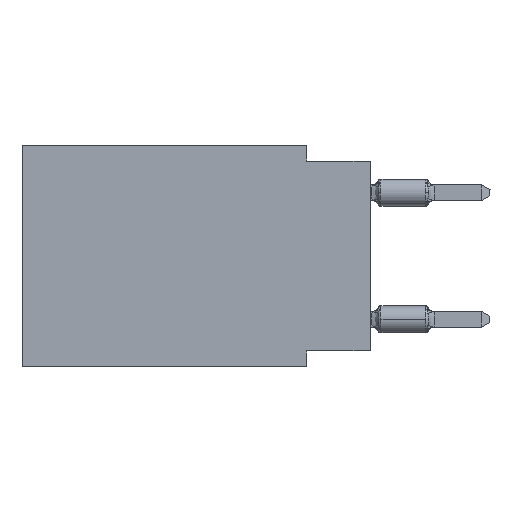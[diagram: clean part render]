
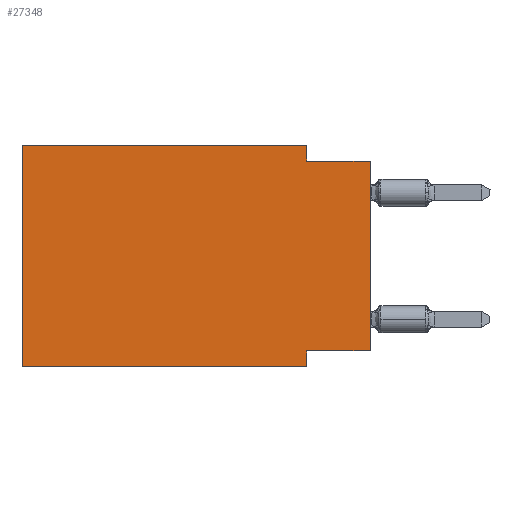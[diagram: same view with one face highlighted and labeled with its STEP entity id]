
A CAD part, left-side view. The second image highlights one B-rep face of the part: STEP entity #27348.
In plain terms, the highlighted planar face has unit normal (-1, 0, 0).
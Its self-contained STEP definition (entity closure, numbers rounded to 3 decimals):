
#410 = CARTESIAN_POINT ( 'NONE',  ( 0., 0., -0.635 ) ) ;
#824 = EDGE_CURVE ( 'NONE', #23125, #20748, #13897, .T. ) ;
#1138 = CARTESIAN_POINT ( 'NONE',  ( 0., 13.97, 0. ) ) ;
#1328 = CARTESIAN_POINT ( 'NONE',  ( 0., 2.54, 0. ) ) ;
#1927 = CARTESIAN_POINT ( 'NONE',  ( 0., 2.54, -0.635 ) ) ;
#3256 = EDGE_CURVE ( 'NONE', #11859, #10257, #14418, .T. ) ;
#3869 = LINE ( 'NONE', #25996, #14602 ) ;
#4015 = VECTOR ( 'NONE', #21537, 1000. ) ;
#4171 = VERTEX_POINT ( 'NONE', #21903 ) ;
#4613 = VECTOR ( 'NONE', #12708, 1000. ) ;
#4654 = CARTESIAN_POINT ( 'NONE',  ( 0., 0., -8.255 ) ) ;
#5295 = VERTEX_POINT ( 'NONE', #4654 ) ;
#5311 = FACE_OUTER_BOUND ( 'NONE', #21102, .T. ) ;
#5463 = LINE ( 'NONE', #19971, #10471 ) ;
#6373 = ORIENTED_EDGE ( 'NONE', *, *, #18525, .F. ) ;
#6732 = CARTESIAN_POINT ( 'NONE',  ( 0., 2.54, 0. ) ) ;
#7529 = DIRECTION ( 'NONE',  ( 0., -1., 0. ) ) ;
#7699 = DIRECTION ( 'NONE',  ( 1., 0., 0. ) ) ;
#8710 = DIRECTION ( 'NONE',  ( 0., 0., 1. ) ) ;
#8904 = LINE ( 'NONE', #17940, #28274 ) ;
#9535 = ORIENTED_EDGE ( 'NONE', *, *, #16182, .F. ) ;
#9789 = VERTEX_POINT ( 'NONE', #6732 ) ;
#10257 = VERTEX_POINT ( 'NONE', #22142 ) ;
#10335 = AXIS2_PLACEMENT_3D ( 'NONE', #1138, #7699, #16742 ) ;
#10471 = VECTOR ( 'NONE', #8710, 1000. ) ;
#10557 = LINE ( 'NONE', #1328, #25677 ) ;
#11704 = EDGE_CURVE ( 'NONE', #9789, #23125, #10557, .T. ) ;
#11859 = VERTEX_POINT ( 'NONE', #20031 ) ;
#12192 = EDGE_CURVE ( 'NONE', #15020, #10257, #13321, .T. ) ;
#12444 = PLANE ( 'NONE',  #10335 ) ;
#12483 = DIRECTION ( 'NONE',  ( 0., 0., -1. ) ) ;
#12708 = DIRECTION ( 'NONE',  ( 0., -1., 0. ) ) ;
#13321 = LINE ( 'NONE', #24443, #18120 ) ;
#13897 = LINE ( 'NONE', #27853, #16418 ) ;
#14418 = LINE ( 'NONE', #19161, #4015 ) ;
#14602 = VECTOR ( 'NONE', #23919, 1000. ) ;
#15020 = VERTEX_POINT ( 'NONE', #22708 ) ;
#15720 = ORIENTED_EDGE ( 'NONE', *, *, #11704, .F. ) ;
#15988 = ORIENTED_EDGE ( 'NONE', *, *, #25869, .F. ) ;
#16182 = EDGE_CURVE ( 'NONE', #5295, #15020, #3869, .T. ) ;
#16418 = VECTOR ( 'NONE', #7529, 1000. ) ;
#16447 = ORIENTED_EDGE ( 'NONE', *, *, #824, .F. ) ;
#16742 = DIRECTION ( 'NONE',  ( 0., 0., -1. ) ) ;
#17940 = CARTESIAN_POINT ( 'NONE',  ( 0., 13.97, 0. ) ) ;
#18120 = VECTOR ( 'NONE', #20418, 1000. ) ;
#18525 = EDGE_CURVE ( 'NONE', #4171, #9789, #24262, .T. ) ;
#18765 = ORIENTED_EDGE ( 'NONE', *, *, #3256, .T. ) ;
#18816 = ORIENTED_EDGE ( 'NONE', *, *, #12192, .F. ) ;
#19161 = CARTESIAN_POINT ( 'NONE',  ( 0., 13.97, -8.89 ) ) ;
#19575 = DIRECTION ( 'NONE',  ( 0., 0., 1. ) ) ;
#19971 = CARTESIAN_POINT ( 'NONE',  ( 0., 0., 0. ) ) ;
#20031 = CARTESIAN_POINT ( 'NONE',  ( 0., 13.97, -8.89 ) ) ;
#20418 = DIRECTION ( 'NONE',  ( 0., 0., -1. ) ) ;
#20748 = VERTEX_POINT ( 'NONE', #410 ) ;
#20939 = EDGE_CURVE ( 'NONE', #5295, #20748, #5463, .T. ) ;
#21102 = EDGE_LOOP ( 'NONE', ( #27754, #16447, #15720, #6373, #15988, #18765, #18816, #9535 ) ) ;
#21537 = DIRECTION ( 'NONE',  ( 0., -1., 0. ) ) ;
#21903 = CARTESIAN_POINT ( 'NONE',  ( 0., 13.97, 0. ) ) ;
#22142 = CARTESIAN_POINT ( 'NONE',  ( 0., 2.54, -8.89 ) ) ;
#22708 = CARTESIAN_POINT ( 'NONE',  ( 0., 2.54, -8.255 ) ) ;
#23125 = VERTEX_POINT ( 'NONE', #1927 ) ;
#23816 = CARTESIAN_POINT ( 'NONE',  ( 0., 13.97, 0. ) ) ;
#23919 = DIRECTION ( 'NONE',  ( 0., 1., 0. ) ) ;
#24262 = LINE ( 'NONE', #23816, #4613 ) ;
#24443 = CARTESIAN_POINT ( 'NONE',  ( 0., 2.54, -8.89 ) ) ;
#25677 = VECTOR ( 'NONE', #12483, 1000. ) ;
#25869 = EDGE_CURVE ( 'NONE', #11859, #4171, #8904, .T. ) ;
#25996 = CARTESIAN_POINT ( 'NONE',  ( 0., 0., -8.255 ) ) ;
#27348 = ADVANCED_FACE ( 'NONE', ( #5311 ), #12444, .F. ) ;
#27754 = ORIENTED_EDGE ( 'NONE', *, *, #20939, .T. ) ;
#27853 = CARTESIAN_POINT ( 'NONE',  ( 0., 0., -0.635 ) ) ;
#28274 = VECTOR ( 'NONE', #19575, 1000. ) ;
